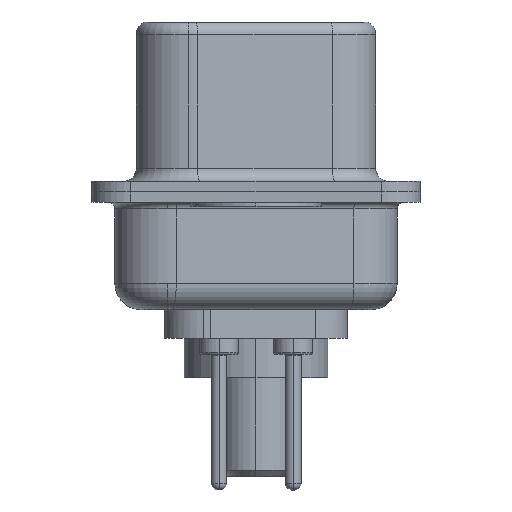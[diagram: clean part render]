
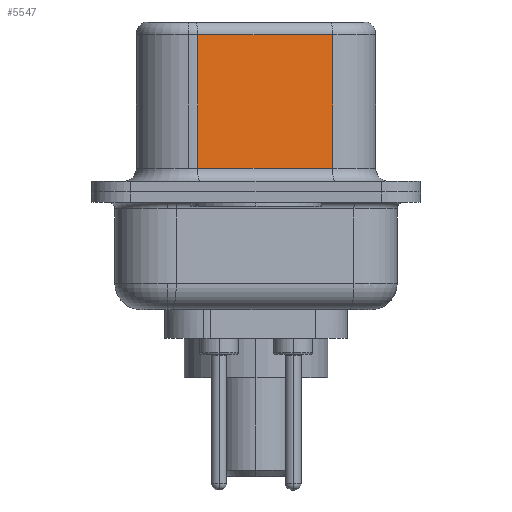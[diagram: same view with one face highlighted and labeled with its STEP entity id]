
A CAD part, left-side view. The second image highlights one B-rep face of the part: STEP entity #5547.
In plain terms, the highlighted planar face has unit normal (-0.985, -0.174, 0).
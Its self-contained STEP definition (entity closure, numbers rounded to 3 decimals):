
#405 = VECTOR ( 'NONE', #2023, 1000. ) ;
#1953 = CARTESIAN_POINT ( 'NONE',  ( 3.655, 2.233, 6.02 ) ) ;
#2023 = DIRECTION ( 'NONE',  ( -0.174, 0.985, 0. ) ) ;
#2144 = CARTESIAN_POINT ( 'NONE',  ( 4.565, -2.927, 6.52 ) ) ;
#2384 = LINE ( 'NONE', #11133, #14873 ) ;
#2613 = CARTESIAN_POINT ( 'NONE',  ( 4.565, -2.927, 0.9 ) ) ;
#2702 = LINE ( 'NONE', #2613, #12025 ) ;
#4024 = ORIENTED_EDGE ( 'NONE', *, *, #12230, .T. ) ;
#4156 = CARTESIAN_POINT ( 'NONE',  ( 4.565, -2.927, 0.9 ) ) ;
#4181 = CARTESIAN_POINT ( 'NONE',  ( 4.565, -2.927, 6.02 ) ) ;
#5008 = PLANE ( 'NONE',  #10969 ) ;
#5049 = VERTEX_POINT ( 'NONE', #1953 ) ;
#5103 = EDGE_LOOP ( 'NONE', ( #10153, #7415, #11625, #4024 ) ) ;
#5547 = ADVANCED_FACE ( 'NONE', ( #10532 ), #5008, .F. ) ;
#6979 = EDGE_CURVE ( 'NONE', #12440, #5049, #7009, .T. ) ;
#7009 = LINE ( 'NONE', #10818, #405 ) ;
#7415 = ORIENTED_EDGE ( 'NONE', *, *, #6979, .T. ) ;
#8138 = CARTESIAN_POINT ( 'NONE',  ( 3.655, 2.233, 0.9 ) ) ;
#8915 = LINE ( 'NONE', #2144, #11305 ) ;
#9518 = VERTEX_POINT ( 'NONE', #8138 ) ;
#10153 = ORIENTED_EDGE ( 'NONE', *, *, #13044, .F. ) ;
#10532 = FACE_OUTER_BOUND ( 'NONE', #5103, .T. ) ;
#10818 = CARTESIAN_POINT ( 'NONE',  ( 4.565, -2.927, 6.02 ) ) ;
#10969 = AXIS2_PLACEMENT_3D ( 'NONE', #13698, #13799, #13855 ) ;
#11133 = CARTESIAN_POINT ( 'NONE',  ( 3.655, 2.233, 6.52 ) ) ;
#11283 = EDGE_CURVE ( 'NONE', #5049, #9518, #2384, .T. ) ;
#11305 = VECTOR ( 'NONE', #11502, 1000. ) ;
#11363 = VERTEX_POINT ( 'NONE', #4156 ) ;
#11502 = DIRECTION ( 'NONE',  ( 0., 0., -1. ) ) ;
#11625 = ORIENTED_EDGE ( 'NONE', *, *, #11283, .T. ) ;
#12025 = VECTOR ( 'NONE', #14370, 1000. ) ;
#12230 = EDGE_CURVE ( 'NONE', #9518, #11363, #2702, .T. ) ;
#12275 = DIRECTION ( 'NONE',  ( 0., 0., -1. ) ) ;
#12440 = VERTEX_POINT ( 'NONE', #4181 ) ;
#13044 = EDGE_CURVE ( 'NONE', #12440, #11363, #8915, .T. ) ;
#13698 = CARTESIAN_POINT ( 'NONE',  ( 4.565, -2.927, 6.52 ) ) ;
#13799 = DIRECTION ( 'NONE',  ( 0.985, 0.174, 0. ) ) ;
#13855 = DIRECTION ( 'NONE',  ( -0.174, 0.985, 0. ) ) ;
#14370 = DIRECTION ( 'NONE',  ( 0.174, -0.985, 0. ) ) ;
#14873 = VECTOR ( 'NONE', #12275, 1000. ) ;
